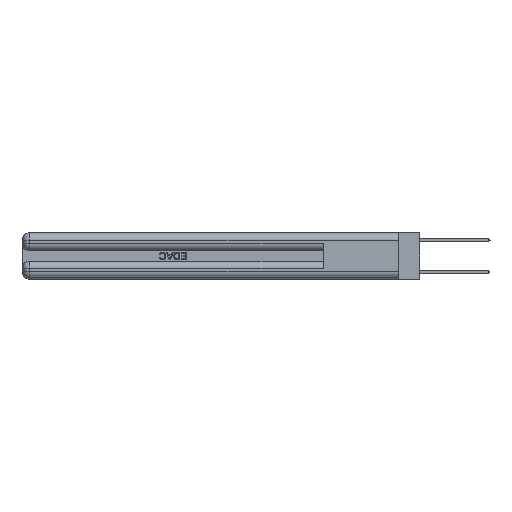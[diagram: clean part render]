
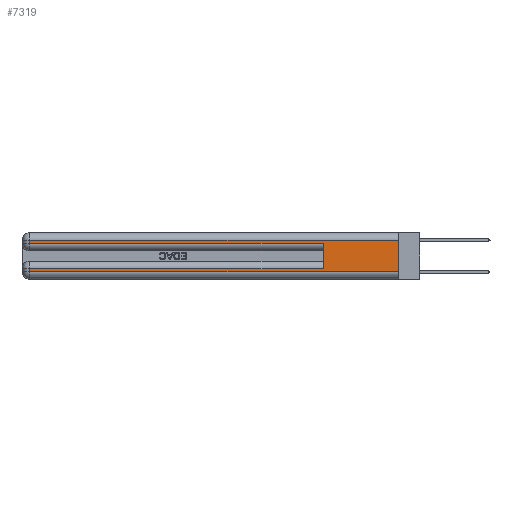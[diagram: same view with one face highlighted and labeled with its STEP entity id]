
A CAD part, left-side view. The second image highlights one B-rep face of the part: STEP entity #7319.
In plain terms, the highlighted planar face has unit normal (-1, 0, 0).
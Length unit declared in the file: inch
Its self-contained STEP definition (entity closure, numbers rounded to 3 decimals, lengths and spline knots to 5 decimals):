
#694 = EDGE_CURVE ( 'NONE', #721, #17517, #18437, .T. ) ;
#721 = VERTEX_POINT ( 'NONE', #32335 ) ;
#904 = EDGE_CURVE ( 'NONE', #8951, #25141, #6748, .T. ) ;
#1074 = ORIENTED_EDGE ( 'NONE', *, *, #17032, .T. ) ;
#1433 = CARTESIAN_POINT ( 'NONE',  ( 0., 2.94, 0.37 ) ) ;
#1912 = LINE ( 'NONE', #27693, #19997 ) ;
#2169 = VECTOR ( 'NONE', #12121, 39.37008 ) ;
#3699 = LINE ( 'NONE', #8343, #9694 ) ;
#3796 = LINE ( 'NONE', #24977, #2169 ) ;
#4845 = VERTEX_POINT ( 'NONE', #18308 ) ;
#4997 = CARTESIAN_POINT ( 'NONE',  ( 0., 0.6, 0.085 ) ) ;
#5452 = LINE ( 'NONE', #11021, #18315 ) ;
#5943 = VECTOR ( 'NONE', #9942, 39.37008 ) ;
#6693 = EDGE_CURVE ( 'NONE', #4845, #25818, #1912, .T. ) ;
#6748 = LINE ( 'NONE', #22783, #5943 ) ;
#6846 = CARTESIAN_POINT ( 'NONE',  ( 0., 0., 0.31 ) ) ;
#7101 = ORIENTED_EDGE ( 'NONE', *, *, #904, .F. ) ;
#7319 = ADVANCED_FACE ( 'NONE', ( #10655 ), #27900, .F. ) ;
#7675 = DIRECTION ( 'NONE',  ( 0., 0., -1. ) ) ;
#7692 = EDGE_LOOP ( 'NONE', ( #11468, #32024, #19154, #19966, #7101, #1074, #28447, #32444 ) ) ;
#8343 = CARTESIAN_POINT ( 'NONE',  ( 0., 0., 0.06 ) ) ;
#8951 = VERTEX_POINT ( 'NONE', #4997 ) ;
#9147 = DIRECTION ( 'NONE',  ( 0., 0., -1. ) ) ;
#9694 = VECTOR ( 'NONE', #23783, 39.37008 ) ;
#9942 = DIRECTION ( 'NONE',  ( 0., 0., 1. ) ) ;
#10655 = FACE_OUTER_BOUND ( 'NONE', #7692, .T. ) ;
#11021 = CARTESIAN_POINT ( 'NONE',  ( 0., 0., 0.285 ) ) ;
#11468 = ORIENTED_EDGE ( 'NONE', *, *, #17078, .F. ) ;
#11535 = CARTESIAN_POINT ( 'NONE',  ( 0., 0., 0.06 ) ) ;
#11560 = VECTOR ( 'NONE', #9147, 39.37008 ) ;
#12121 = DIRECTION ( 'NONE',  ( 0., 0., -1. ) ) ;
#12464 = CARTESIAN_POINT ( 'NONE',  ( 0., 0., 0.37 ) ) ;
#13630 = DIRECTION ( 'NONE',  ( 0., -1., 0. ) ) ;
#14225 = EDGE_CURVE ( 'NONE', #25818, #24589, #3699, .T. ) ;
#14525 = LINE ( 'NONE', #15164, #19756 ) ;
#15054 = DIRECTION ( 'NONE',  ( 1., 0., 0. ) ) ;
#15111 = AXIS2_PLACEMENT_3D ( 'NONE', #12464, #15054, #33048 ) ;
#15164 = CARTESIAN_POINT ( 'NONE',  ( 0., 0., 0.31 ) ) ;
#15366 = EDGE_CURVE ( 'NONE', #29153, #721, #14525, .T. ) ;
#17032 = EDGE_CURVE ( 'NONE', #8951, #4845, #25102, .T. ) ;
#17078 = EDGE_CURVE ( 'NONE', #29153, #24589, #3796, .T. ) ;
#17517 = VERTEX_POINT ( 'NONE', #19695 ) ;
#18308 = CARTESIAN_POINT ( 'NONE',  ( 0., 2.94, 0.085 ) ) ;
#18315 = VECTOR ( 'NONE', #13630, 39.37008 ) ;
#18437 = LINE ( 'NONE', #1433, #11560 ) ;
#18772 = CARTESIAN_POINT ( 'NONE',  ( 0., 2.94, 0.06 ) ) ;
#19154 = ORIENTED_EDGE ( 'NONE', *, *, #694, .T. ) ;
#19695 = CARTESIAN_POINT ( 'NONE',  ( 0., 2.94, 0.285 ) ) ;
#19756 = VECTOR ( 'NONE', #28010, 39.37008 ) ;
#19966 = ORIENTED_EDGE ( 'NONE', *, *, #31904, .T. ) ;
#19997 = VECTOR ( 'NONE', #7675, 39.37008 ) ;
#22783 = CARTESIAN_POINT ( 'NONE',  ( 0., 0.6, 0.145 ) ) ;
#23489 = VECTOR ( 'NONE', #24744, 39.37008 ) ;
#23783 = DIRECTION ( 'NONE',  ( 0., -1., 0. ) ) ;
#24589 = VERTEX_POINT ( 'NONE', #11535 ) ;
#24744 = DIRECTION ( 'NONE',  ( 0., 1., 0. ) ) ;
#24977 = CARTESIAN_POINT ( 'NONE',  ( 0., 0., 0.37 ) ) ;
#25102 = LINE ( 'NONE', #27331, #23489 ) ;
#25141 = VERTEX_POINT ( 'NONE', #31871 ) ;
#25818 = VERTEX_POINT ( 'NONE', #18772 ) ;
#27331 = CARTESIAN_POINT ( 'NONE',  ( 0., 0., 0.085 ) ) ;
#27693 = CARTESIAN_POINT ( 'NONE',  ( 0., 2.94, 0.37 ) ) ;
#27900 = PLANE ( 'NONE',  #15111 ) ;
#28010 = DIRECTION ( 'NONE',  ( 0., 1., 0. ) ) ;
#28447 = ORIENTED_EDGE ( 'NONE', *, *, #6693, .T. ) ;
#29153 = VERTEX_POINT ( 'NONE', #6846 ) ;
#31871 = CARTESIAN_POINT ( 'NONE',  ( 0., 0.6, 0.285 ) ) ;
#31904 = EDGE_CURVE ( 'NONE', #17517, #25141, #5452, .T. ) ;
#32024 = ORIENTED_EDGE ( 'NONE', *, *, #15366, .T. ) ;
#32335 = CARTESIAN_POINT ( 'NONE',  ( 0., 2.94, 0.31 ) ) ;
#32444 = ORIENTED_EDGE ( 'NONE', *, *, #14225, .T. ) ;
#33048 = DIRECTION ( 'NONE',  ( 0., 0., -1. ) ) ;
